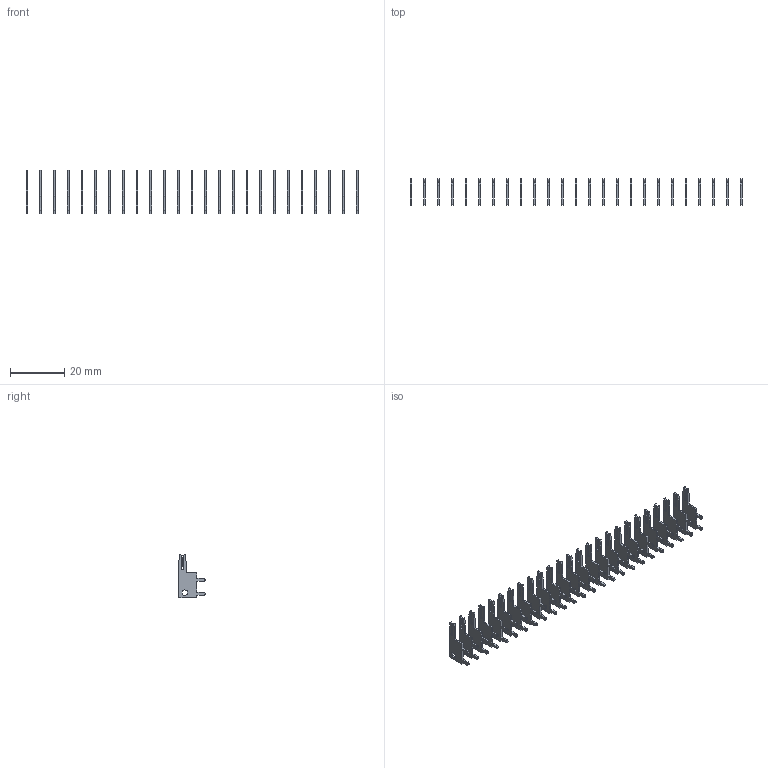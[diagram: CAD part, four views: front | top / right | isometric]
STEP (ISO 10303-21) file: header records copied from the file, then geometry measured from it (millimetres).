
FILE_DESCRIPTION (( 'STEP AP203' ), '1' );
FILE_NAME ('105-025-201-200.STEP', '2020-04-07T23:10:41', ( '' ), ( '' ), 'SwSTEP 2.0', 'SolidWorks 2016', '' );
FILE_SCHEMA (( 'CONFIG_CONTROL_DESIGN' ));
Length unit declared in the file: inch
Products named in the file (2): 100-290-001_100-290-201; 105-025-201-200
Assembly tree (25 placements, depth 2):
  105-025-201-200
    100-290-001_100-290-201  x25
Bounding box: 122.56 x 9.7 x 15.88 mm (x, y, z)
Volume: 1231 mm3; surface area: 5023.5 mm2
Topology: 25 solids, 25 shells, 875 faces, 2475 edges, 1650 vertices
Faces by surface type: plane 625, cylinder 250
Entity records: 2105 total; most frequent: DIRECTION 241, CARTESIAN_POINT 240, ORIENTED_EDGE 198, EDGE_CURVE 99, AXIS2_PLACEMENT_3D 83, VECTOR 75, LINE 75, VERTEX_POINT 66
